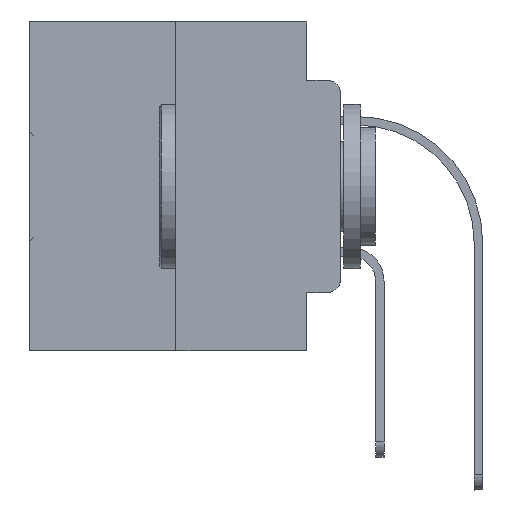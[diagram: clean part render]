
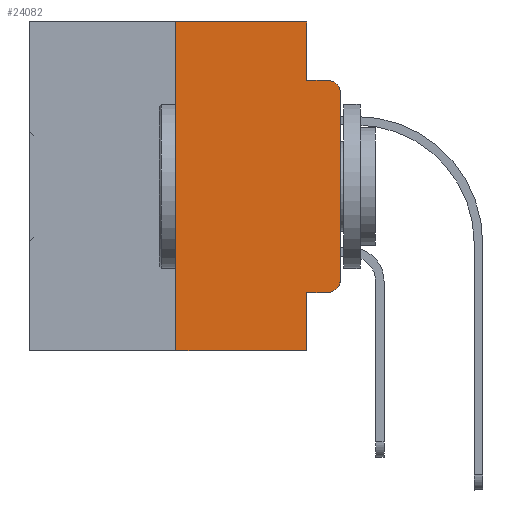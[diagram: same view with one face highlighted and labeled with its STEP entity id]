
A CAD part, left-side view. The second image highlights one B-rep face of the part: STEP entity #24082.
In plain terms, the highlighted planar face has unit normal (-1, 0, 0).
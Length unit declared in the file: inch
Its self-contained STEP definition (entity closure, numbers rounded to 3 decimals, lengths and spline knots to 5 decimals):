
#125 = LINE ( 'NONE', #22864, #2595 ) ;
#191 = CARTESIAN_POINT ( 'NONE',  ( 0., 0.473, 0. ) ) ;
#330 = DIRECTION ( 'NONE',  ( -1., 0., 0. ) ) ;
#498 = DIRECTION ( 'NONE',  ( 0., 0., -1. ) ) ;
#847 = CARTESIAN_POINT ( 'NONE',  ( 0., 0.02, -0.1085 ) ) ;
#852 = EDGE_CURVE ( 'NONE', #32891, #2160, #10955, .T. ) ;
#2160 = VERTEX_POINT ( 'NONE', #14866 ) ;
#2210 = DIRECTION ( 'NONE',  ( 0., -1., 0. ) ) ;
#2368 = EDGE_CURVE ( 'NONE', #16433, #27127, #10812, .T. ) ;
#2595 = VECTOR ( 'NONE', #5550, 39.37008 ) ;
#3671 = CARTESIAN_POINT ( 'NONE',  ( 0., 0.02, -0.3915 ) ) ;
#3722 = DIRECTION ( 'NONE',  ( 0., -1., 0. ) ) ;
#4889 = VECTOR ( 'NONE', #3722, 39.37008 ) ;
#5161 = DIRECTION ( 'NONE',  ( 1., 0., 0. ) ) ;
#5489 = ORIENTED_EDGE ( 'NONE', *, *, #2368, .T. ) ;
#5550 = DIRECTION ( 'NONE',  ( 0., 0., 1. ) ) ;
#6085 = CARTESIAN_POINT ( 'NONE',  ( 0., 0.473, -0.5 ) ) ;
#6460 = CARTESIAN_POINT ( 'NONE',  ( 0., 0.25, 0. ) ) ;
#6484 = CIRCLE ( 'NONE', #33839, 0.02 ) ;
#6896 = ORIENTED_EDGE ( 'NONE', *, *, #22664, .F. ) ;
#7070 = EDGE_CURVE ( 'NONE', #33829, #15255, #32357, .T. ) ;
#8013 = CARTESIAN_POINT ( 'NONE',  ( 0., 0.051, -0.4115 ) ) ;
#8653 = VECTOR ( 'NONE', #19670, 39.37008 ) ;
#8959 = ORIENTED_EDGE ( 'NONE', *, *, #32588, .T. ) ;
#9633 = AXIS2_PLACEMENT_3D ( 'NONE', #3671, #330, #498 ) ;
#10204 = CARTESIAN_POINT ( 'NONE',  ( 0., 0.051, -0.4115 ) ) ;
#10812 = CIRCLE ( 'NONE', #9633, 0.02 ) ;
#10955 = LINE ( 'NONE', #28259, #12927 ) ;
#12927 = VECTOR ( 'NONE', #2210, 39.37008 ) ;
#14748 = CARTESIAN_POINT ( 'NONE',  ( 0., 0.051, 0. ) ) ;
#14866 = CARTESIAN_POINT ( 'NONE',  ( 0., 0.02, -0.0885 ) ) ;
#14881 = EDGE_CURVE ( 'NONE', #27422, #20472, #22470, .T. ) ;
#15255 = VERTEX_POINT ( 'NONE', #16297 ) ;
#15367 = DIRECTION ( 'NONE',  ( -1., 0., 0. ) ) ;
#15620 = LINE ( 'NONE', #10204, #4889 ) ;
#16297 = CARTESIAN_POINT ( 'NONE',  ( 0., 0.25, 0. ) ) ;
#16328 = CARTESIAN_POINT ( 'NONE',  ( 0., 0.473, 0. ) ) ;
#16433 = VERTEX_POINT ( 'NONE', #36226 ) ;
#16833 = CARTESIAN_POINT ( 'NONE',  ( 0., 0., -0.3915 ) ) ;
#18340 = ORIENTED_EDGE ( 'NONE', *, *, #21835, .F. ) ;
#18884 = EDGE_CURVE ( 'NONE', #27127, #22907, #125, .T. ) ;
#19218 = CARTESIAN_POINT ( 'NONE',  ( 0., 0., -0.1085 ) ) ;
#19670 = DIRECTION ( 'NONE',  ( 0., 0., -1. ) ) ;
#20472 = VERTEX_POINT ( 'NONE', #23422 ) ;
#21270 = VERTEX_POINT ( 'NONE', #31885 ) ;
#21835 = EDGE_CURVE ( 'NONE', #15255, #21270, #31673, .T. ) ;
#22059 = CARTESIAN_POINT ( 'NONE',  ( 0., 0.051, -0.0885 ) ) ;
#22470 = LINE ( 'NONE', #25280, #8653 ) ;
#22664 = EDGE_CURVE ( 'NONE', #21270, #32891, #28890, .T. ) ;
#22864 = CARTESIAN_POINT ( 'NONE',  ( 0., 0., 0. ) ) ;
#22907 = VERTEX_POINT ( 'NONE', #19218 ) ;
#23422 = CARTESIAN_POINT ( 'NONE',  ( 0., 0.051, -0.5 ) ) ;
#23514 = ORIENTED_EDGE ( 'NONE', *, *, #18884, .T. ) ;
#24082 = ADVANCED_FACE ( 'NONE', ( #25444 ), #30471, .F. ) ;
#24970 = ORIENTED_EDGE ( 'NONE', *, *, #35030, .T. ) ;
#25280 = CARTESIAN_POINT ( 'NONE',  ( 0., 0.051, 0. ) ) ;
#25444 = FACE_OUTER_BOUND ( 'NONE', #34544, .T. ) ;
#25479 = VECTOR ( 'NONE', #32530, 39.37008 ) ;
#25642 = LINE ( 'NONE', #6085, #34552 ) ;
#26008 = DIRECTION ( 'NONE',  ( 0., 0., -1. ) ) ;
#26318 = DIRECTION ( 'NONE',  ( 0., 0., -1. ) ) ;
#27127 = VERTEX_POINT ( 'NONE', #16833 ) ;
#27145 = AXIS2_PLACEMENT_3D ( 'NONE', #16328, #5161, #28392 ) ;
#27422 = VERTEX_POINT ( 'NONE', #8013 ) ;
#28259 = CARTESIAN_POINT ( 'NONE',  ( 0., 0.051, -0.0885 ) ) ;
#28392 = DIRECTION ( 'NONE',  ( 0., 0., -1. ) ) ;
#28890 = LINE ( 'NONE', #14748, #31312 ) ;
#29041 = EDGE_CURVE ( 'NONE', #27422, #16433, #15620, .T. ) ;
#29247 = ORIENTED_EDGE ( 'NONE', *, *, #7070, .F. ) ;
#29515 = CARTESIAN_POINT ( 'NONE',  ( 0., 0.25, -0.5 ) ) ;
#29652 = ORIENTED_EDGE ( 'NONE', *, *, #14881, .F. ) ;
#30471 = PLANE ( 'NONE',  #27145 ) ;
#31237 = DIRECTION ( 'NONE',  ( 0., -1., 0. ) ) ;
#31269 = VECTOR ( 'NONE', #34829, 39.37008 ) ;
#31312 = VECTOR ( 'NONE', #26318, 39.37008 ) ;
#31453 = ORIENTED_EDGE ( 'NONE', *, *, #29041, .T. ) ;
#31673 = LINE ( 'NONE', #191, #31269 ) ;
#31885 = CARTESIAN_POINT ( 'NONE',  ( 0., 0.051, 0. ) ) ;
#32357 = LINE ( 'NONE', #6460, #25479 ) ;
#32530 = DIRECTION ( 'NONE',  ( 0., 0., 1. ) ) ;
#32588 = EDGE_CURVE ( 'NONE', #22907, #2160, #6484, .T. ) ;
#32891 = VERTEX_POINT ( 'NONE', #22059 ) ;
#33829 = VERTEX_POINT ( 'NONE', #29515 ) ;
#33839 = AXIS2_PLACEMENT_3D ( 'NONE', #847, #15367, #26008 ) ;
#34544 = EDGE_LOOP ( 'NONE', ( #23514, #8959, #36042, #6896, #18340, #29247, #24970, #29652, #31453, #5489 ) ) ;
#34552 = VECTOR ( 'NONE', #31237, 39.37008 ) ;
#34829 = DIRECTION ( 'NONE',  ( 0., -1., 0. ) ) ;
#35030 = EDGE_CURVE ( 'NONE', #33829, #20472, #25642, .T. ) ;
#36042 = ORIENTED_EDGE ( 'NONE', *, *, #852, .F. ) ;
#36226 = CARTESIAN_POINT ( 'NONE',  ( 0., 0.02, -0.4115 ) ) ;
